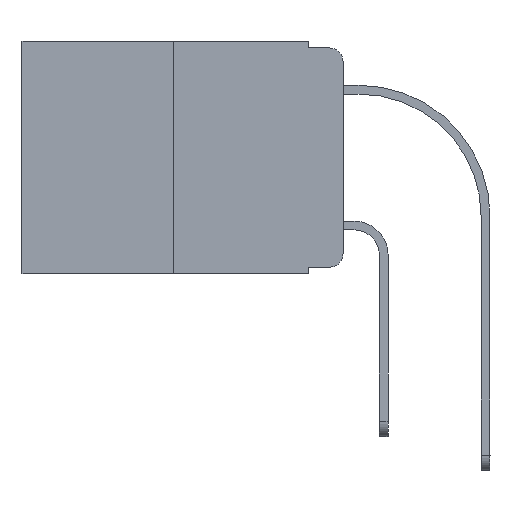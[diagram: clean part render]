
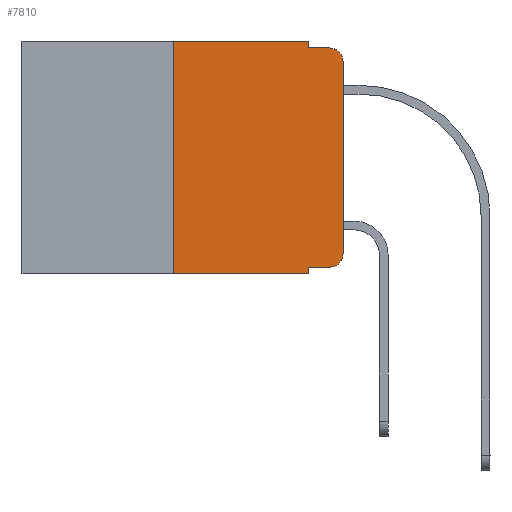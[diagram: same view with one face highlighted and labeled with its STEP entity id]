
A CAD part, left-side view. The second image highlights one B-rep face of the part: STEP entity #7810.
In plain terms, the highlighted planar face has unit normal (-1, 0, 0).
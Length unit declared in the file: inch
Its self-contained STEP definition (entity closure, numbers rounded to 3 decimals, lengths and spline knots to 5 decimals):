
#46 = ORIENTED_EDGE ( 'NONE', *, *, #1830, .F. ) ;
#90 = LINE ( 'NONE', #16200, #2656 ) ;
#126 = CARTESIAN_POINT ( 'NONE',  ( 0., 0.051, -0.333 ) ) ;
#143 = ORIENTED_EDGE ( 'NONE', *, *, #5997, .T. ) ;
#500 = CARTESIAN_POINT ( 'NONE',  ( 0., 0.051, -0.343 ) ) ;
#711 = EDGE_CURVE ( 'NONE', #4584, #18251, #5948, .T. ) ;
#789 = ORIENTED_EDGE ( 'NONE', *, *, #1771, .F. ) ;
#1511 = VECTOR ( 'NONE', #6149, 39.37008 ) ;
#1672 = VERTEX_POINT ( 'NONE', #13424 ) ;
#1771 = EDGE_CURVE ( 'NONE', #11572, #8818, #10507, .T. ) ;
#1830 = EDGE_CURVE ( 'NONE', #16786, #2024, #9110, .T. ) ;
#2024 = VERTEX_POINT ( 'NONE', #500 ) ;
#2656 = VECTOR ( 'NONE', #3205, 39.37008 ) ;
#3205 = DIRECTION ( 'NONE',  ( 0., -1., 0. ) ) ;
#3426 = EDGE_CURVE ( 'NONE', #8818, #14746, #18430, .T. ) ;
#3538 = EDGE_CURVE ( 'NONE', #14746, #14166, #20451, .T. ) ;
#3861 = ORIENTED_EDGE ( 'NONE', *, *, #711, .T. ) ;
#4274 = DIRECTION ( 'NONE',  ( 0., -1., 0. ) ) ;
#4584 = VERTEX_POINT ( 'NONE', #16827 ) ;
#5266 = EDGE_CURVE ( 'NONE', #1672, #21095, #16474, .T. ) ;
#5676 = CARTESIAN_POINT ( 'NONE',  ( 0., 0.02, -0.03 ) ) ;
#5948 = CIRCLE ( 'NONE', #14526, 0.02 ) ;
#5997 = EDGE_CURVE ( 'NONE', #11572, #2024, #15652, .T. ) ;
#6149 = DIRECTION ( 'NONE',  ( 0., 0., 1. ) ) ;
#7308 = CARTESIAN_POINT ( 'NONE',  ( 0., 0.25, 0. ) ) ;
#7810 = ADVANCED_FACE ( 'NONE', ( #11314 ), #12819, .F. ) ;
#7826 = DIRECTION ( 'NONE',  ( 0., 0., -1. ) ) ;
#7936 = EDGE_CURVE ( 'NONE', #21095, #4584, #9266, .T. ) ;
#7990 = CARTESIAN_POINT ( 'NONE',  ( 0., 0.02, -0.313 ) ) ;
#8818 = VERTEX_POINT ( 'NONE', #10822 ) ;
#9088 = CARTESIAN_POINT ( 'NONE',  ( 0., 0.051, 0. ) ) ;
#9110 = LINE ( 'NONE', #14167, #20166 ) ;
#9266 = LINE ( 'NONE', #10865, #1511 ) ;
#9554 = VECTOR ( 'NONE', #13014, 39.37008 ) ;
#9900 = VECTOR ( 'NONE', #20689, 39.37008 ) ;
#10004 = ORIENTED_EDGE ( 'NONE', *, *, #5266, .T. ) ;
#10507 = LINE ( 'NONE', #7308, #9900 ) ;
#10822 = CARTESIAN_POINT ( 'NONE',  ( 0., 0.25, 0. ) ) ;
#10865 = CARTESIAN_POINT ( 'NONE',  ( 0., 0., 0. ) ) ;
#11022 = VECTOR ( 'NONE', #4274, 39.37008 ) ;
#11202 = DIRECTION ( 'NONE',  ( 0., 0., -1. ) ) ;
#11314 = FACE_OUTER_BOUND ( 'NONE', #13171, .T. ) ;
#11572 = VERTEX_POINT ( 'NONE', #18912 ) ;
#11613 = LINE ( 'NONE', #126, #9554 ) ;
#12221 = DIRECTION ( 'NONE',  ( -1., 0., 0. ) ) ;
#12435 = CARTESIAN_POINT ( 'NONE',  ( 0., 0.473, -0.343 ) ) ;
#12437 = ORIENTED_EDGE ( 'NONE', *, *, #13659, .F. ) ;
#12501 = DIRECTION ( 'NONE',  ( 0., 0., -1. ) ) ;
#12819 = PLANE ( 'NONE',  #14195 ) ;
#12916 = CARTESIAN_POINT ( 'NONE',  ( 0., 0.473, 0. ) ) ;
#13014 = DIRECTION ( 'NONE',  ( 0., -1., 0. ) ) ;
#13171 = EDGE_LOOP ( 'NONE', ( #17661, #3861, #12437, #13771, #20771, #789, #143, #46, #19556, #10004 ) ) ;
#13211 = CARTESIAN_POINT ( 'NONE',  ( 0., 0.051, -0.333 ) ) ;
#13424 = CARTESIAN_POINT ( 'NONE',  ( 0., 0.02, -0.333 ) ) ;
#13659 = EDGE_CURVE ( 'NONE', #14166, #18251, #90, .T. ) ;
#13714 = DIRECTION ( 'NONE',  ( 0., 0., -1. ) ) ;
#13771 = ORIENTED_EDGE ( 'NONE', *, *, #3538, .F. ) ;
#14166 = VERTEX_POINT ( 'NONE', #17670 ) ;
#14167 = CARTESIAN_POINT ( 'NONE',  ( 0., 0.051, 0. ) ) ;
#14195 = AXIS2_PLACEMENT_3D ( 'NONE', #12916, #17856, #11202 ) ;
#14526 = AXIS2_PLACEMENT_3D ( 'NONE', #5676, #12221, #18773 ) ;
#14538 = DIRECTION ( 'NONE',  ( -1., 0., 0. ) ) ;
#14717 = VECTOR ( 'NONE', #13714, 39.37008 ) ;
#14746 = VERTEX_POINT ( 'NONE', #14865 ) ;
#14865 = CARTESIAN_POINT ( 'NONE',  ( 0., 0.051, 0. ) ) ;
#15190 = CARTESIAN_POINT ( 'NONE',  ( 0., 0.02, -0.01 ) ) ;
#15447 = VECTOR ( 'NONE', #16923, 39.37008 ) ;
#15652 = LINE ( 'NONE', #12435, #11022 ) ;
#16200 = CARTESIAN_POINT ( 'NONE',  ( 0., 0.051, -0.01 ) ) ;
#16458 = AXIS2_PLACEMENT_3D ( 'NONE', #7990, #14538, #12501 ) ;
#16474 = CIRCLE ( 'NONE', #16458, 0.02 ) ;
#16614 = CARTESIAN_POINT ( 'NONE',  ( 0., 0.473, 0. ) ) ;
#16786 = VERTEX_POINT ( 'NONE', #13211 ) ;
#16827 = CARTESIAN_POINT ( 'NONE',  ( 0., 0., -0.03 ) ) ;
#16923 = DIRECTION ( 'NONE',  ( 0., -1., 0. ) ) ;
#17661 = ORIENTED_EDGE ( 'NONE', *, *, #7936, .T. ) ;
#17670 = CARTESIAN_POINT ( 'NONE',  ( 0., 0.051, -0.01 ) ) ;
#17856 = DIRECTION ( 'NONE',  ( 1., 0., 0. ) ) ;
#18251 = VERTEX_POINT ( 'NONE', #15190 ) ;
#18430 = LINE ( 'NONE', #16614, #15447 ) ;
#18773 = DIRECTION ( 'NONE',  ( 0., 0., -1. ) ) ;
#18912 = CARTESIAN_POINT ( 'NONE',  ( 0., 0.25, -0.343 ) ) ;
#19089 = CARTESIAN_POINT ( 'NONE',  ( 0., 0., -0.313 ) ) ;
#19556 = ORIENTED_EDGE ( 'NONE', *, *, #20958, .T. ) ;
#20166 = VECTOR ( 'NONE', #7826, 39.37008 ) ;
#20451 = LINE ( 'NONE', #9088, #14717 ) ;
#20689 = DIRECTION ( 'NONE',  ( 0., 0., 1. ) ) ;
#20771 = ORIENTED_EDGE ( 'NONE', *, *, #3426, .F. ) ;
#20958 = EDGE_CURVE ( 'NONE', #16786, #1672, #11613, .T. ) ;
#21095 = VERTEX_POINT ( 'NONE', #19089 ) ;
